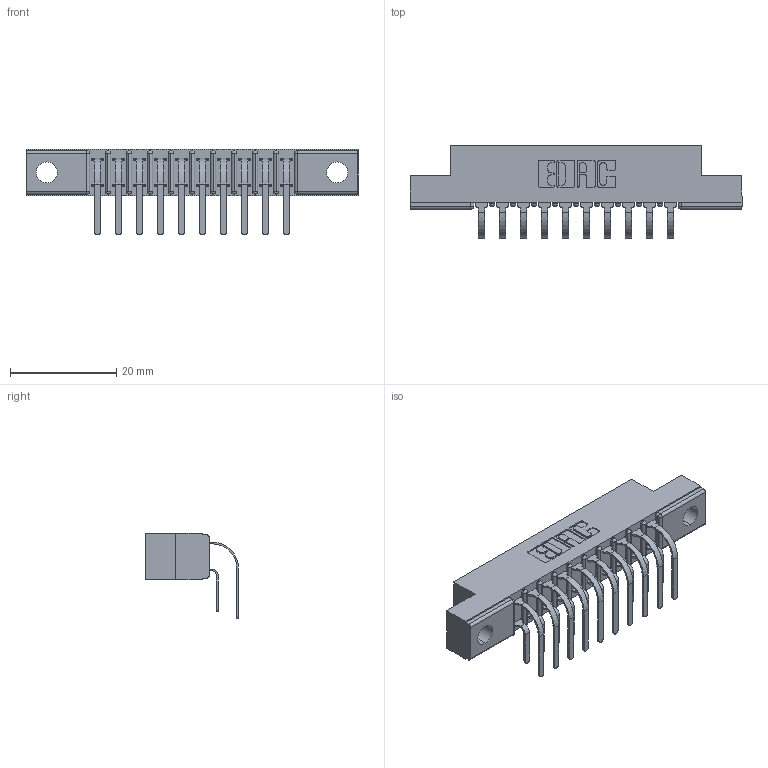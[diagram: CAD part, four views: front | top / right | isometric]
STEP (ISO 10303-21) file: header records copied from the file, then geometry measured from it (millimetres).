
FILE_DESCRIPTION (( 'STEP AP203' ), '1' );
FILE_NAME ('357-020-459-204.STEP', '2022-07-08T01:00:32', ( '' ), ( '' ), 'SwSTEP 2.0', 'SolidWorks 2020', '' );
FILE_SCHEMA (( 'CONFIG_CONTROL_DESIGN' ));
Length unit declared in the file: inch
Products named in the file (4): 307-290-001_559 - 2 (Single); 357-020-459-204; 307 Part_.156 Dia Mounting Holes; 307-290-001_558 559 - 1 (Single)
Assembly tree (21 placements, depth 2):
  357-020-459-204
    307 Part_.156 Dia Mounting Holes
    307-290-001_558 559 - 1 (Single)  x10
    307-290-001_559 - 2 (Single)  x10
Bounding box: 62.64 x 17.51 x 16.08 mm (x, y, z)
Volume: 4067.7 mm3; surface area: 6865.7 mm2
Topology: 21 solids, 21 shells, 1143 faces, 3199 edges, 2074 vertices
Faces by surface type: plane 744, cylinder 377, sphere 22
Entity records: 14703 total; most frequent: CARTESIAN_POINT 2422, ORIENTED_EDGE 2394, DIRECTION 2377, EDGE_CURVE 1197, LINE 911, VECTOR 911, VERTEX_POINT 778, AXIS2_PLACEMENT_3D 733
